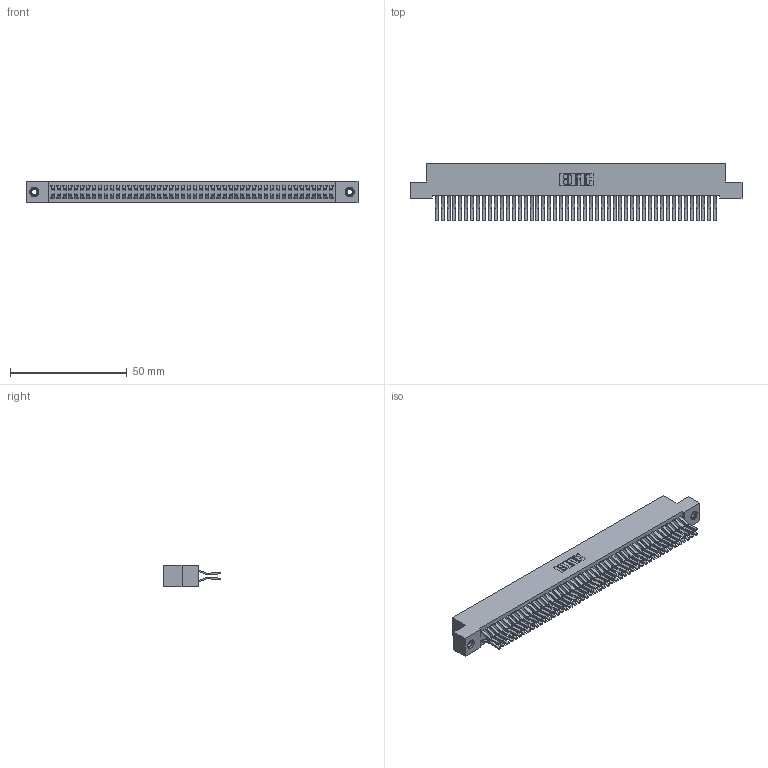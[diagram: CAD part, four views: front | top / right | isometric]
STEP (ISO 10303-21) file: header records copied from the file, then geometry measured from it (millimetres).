
FILE_DESCRIPTION (( 'STEP AP203' ), '1' );
FILE_NAME ('342-096-560-207.STEP', '2019-10-04T16:25:43', ( '' ), ( '' ), 'SwSTEP 2.0', 'SolidWorks 2016', '' );
FILE_SCHEMA (( 'CONFIG_CONTROL_DESIGN' ));
Length unit declared in the file: inch
Products named in the file (4): 345-292-001_560 Tail; 345-250-001_345-250-005-103; 342-096-560-207; 342 Part_TI
Assembly tree (99 placements, depth 2):
  342-096-560-207
    342 Part_TI
    345-292-001_560 Tail  x96
    345-250-001_345-250-005-103  x2
Bounding box: 142.24 x 24.78 x 9.4 mm (x, y, z)
Volume: 13426.2 mm3; surface area: 23539.5 mm2
Topology: 99 solids, 99 shells, 5354 faces, 15891 edges, 10458 vertices
Faces by surface type: plane 3554, cylinder 1784, cone 12, torus 4
Entity records: 31246 total; most frequent: CARTESIAN_POINT 5153, ORIENTED_EDGE 5082, DIRECTION 4427, EDGE_CURVE 2541, VECTOR 2389, LINE 2389, VERTEX_POINT 1688, AXIS2_PLACEMENT_3D 1019
